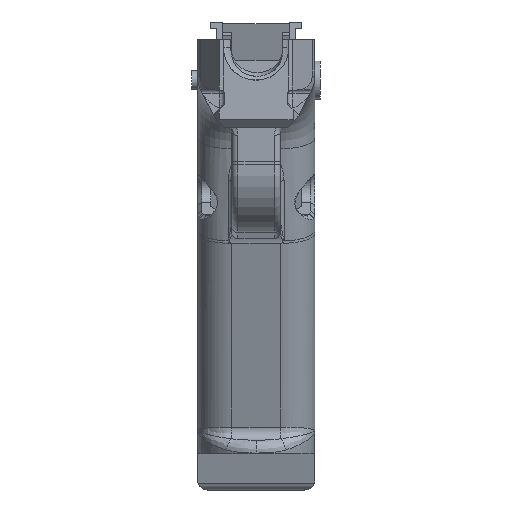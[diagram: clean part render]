
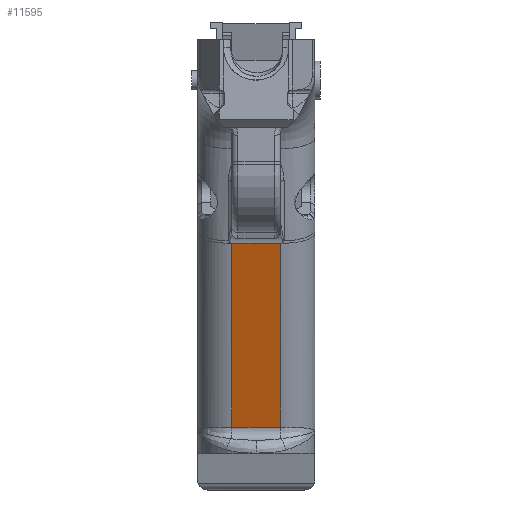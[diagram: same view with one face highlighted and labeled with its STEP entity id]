
A CAD part, front view. The second image highlights one B-rep face of the part: STEP entity #11595.
In plain terms, the highlighted planar face has unit normal (0, -0.947, -0.322).
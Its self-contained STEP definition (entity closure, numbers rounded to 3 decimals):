
#1336=FACE_OUTER_BOUND('',#1979,.T.);
#1979=EDGE_LOOP('',(#9772,#9773,#9774,#9775));
#2867=LINE('',#19605,#4046);
#3007=LINE('',#22061,#4186);
#3008=LINE('',#22069,#4187);
#3009=LINE('',#22070,#4188);
#4046=VECTOR('',#14391,10.);
#4186=VECTOR('',#14771,10.);
#4187=VECTOR('',#14774,10.);
#4188=VECTOR('',#14775,10.);
#5184=VERTEX_POINT('',#19598);
#5185=VERTEX_POINT('',#19604);
#5365=VERTEX_POINT('',#22053);
#5366=VERTEX_POINT('',#22060);
#6637=EDGE_CURVE('',#5184,#5185,#2867,.T.);
#6919=EDGE_CURVE('',#5365,#5366,#3007,.T.);
#6921=EDGE_CURVE('',#5366,#5184,#3008,.T.);
#6922=EDGE_CURVE('',#5185,#5365,#3009,.T.);
#9772=ORIENTED_EDGE('',*,*,#6637,.F.);
#9773=ORIENTED_EDGE('',*,*,#6921,.F.);
#9774=ORIENTED_EDGE('',*,*,#6919,.F.);
#9775=ORIENTED_EDGE('',*,*,#6922,.F.);
#11027=PLANE('',#12459);
#11595=ADVANCED_FACE('',(#1336),#11027,.T.);
#12459=AXIS2_PLACEMENT_3D('',#22068,#14772,#14773);
#14391=DIRECTION('',(-1.,0.,0.));
#14771=DIRECTION('',(1.,0.,0.));
#14772=DIRECTION('center_axis',(0.,-0.947,-0.322));
#14773=DIRECTION('ref_axis',(0.,0.322,-0.947));
#14774=DIRECTION('',(0.,0.322,-0.947));
#14775=DIRECTION('',(0.,-0.322,0.947));
#19598=CARTESIAN_POINT('',(-2.118,-62.644,-85.79));
#19604=CARTESIAN_POINT('',(-14.218,-62.644,-85.79));
#19605=CARTESIAN_POINT('',(-15.418,-62.644,-85.79));
#22053=CARTESIAN_POINT('',(-14.218,-78.109,-40.345));
#22060=CARTESIAN_POINT('',(-2.118,-78.109,-40.345));
#22061=CARTESIAN_POINT('',(0.,-78.109,-40.345));
#22068=CARTESIAN_POINT('Origin',(-22.668,-78.109,-40.345));
#22069=CARTESIAN_POINT('',(-2.118,-83.303,-25.083));
#22070=CARTESIAN_POINT('',(-14.218,-83.303,-25.083));
